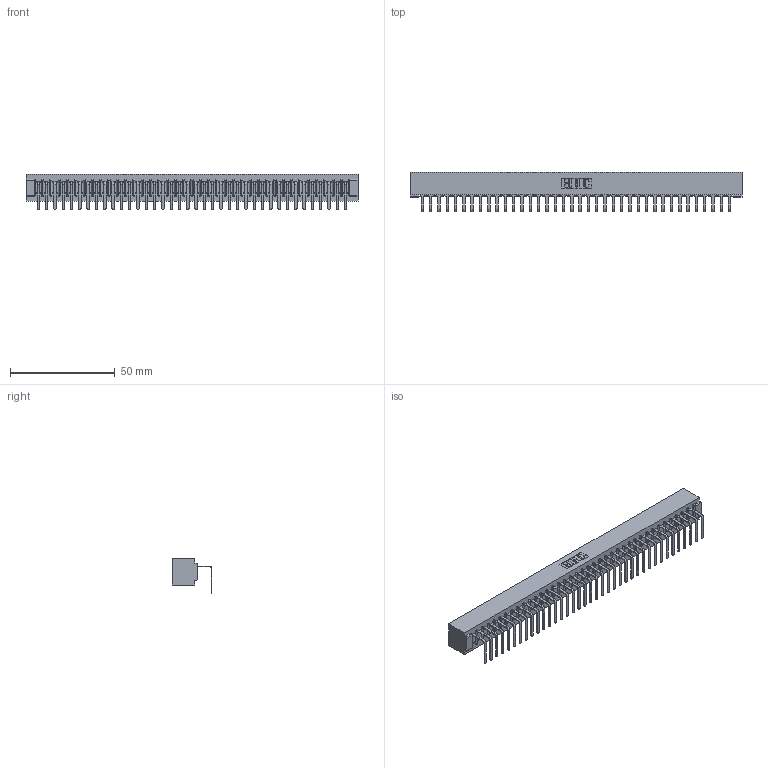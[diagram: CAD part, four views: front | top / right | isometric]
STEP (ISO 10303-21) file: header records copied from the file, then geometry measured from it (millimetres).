
FILE_DESCRIPTION (( 'STEP AP203' ), '1' );
FILE_NAME ('307-038-558-101.STEP', '2019-09-05T14:48:10', ( '' ), ( '' ), 'SwSTEP 2.0', 'SolidWorks 2016', '' );
FILE_SCHEMA (( 'CONFIG_CONTROL_DESIGN' ));
Length unit declared in the file: inch
Products named in the file (3): 307-290-001_558 - 2 (Single); 307-038-558-101; 307 Part_No Mounting Lugs
Assembly tree (39 placements, depth 2):
  307-038-558-101
    307 Part_No Mounting Lugs
    307-290-001_558 - 2 (Single)  x38
Bounding box: 158.45 x 18.96 x 16.8 mm (x, y, z)
Volume: 17107.4 mm3; surface area: 19328.5 mm2
Topology: 39 solids, 39 shells, 2429 faces, 6911 edges, 4450 vertices
Faces by surface type: plane 1548, cylinder 803, sphere 78
Entity records: 32896 total; most frequent: CARTESIAN_POINT 5540, ORIENTED_EDGE 5526, DIRECTION 5389, EDGE_CURVE 2763, VECTOR 2119, LINE 2119, VERTEX_POINT 1786, AXIS2_PLACEMENT_3D 1635
